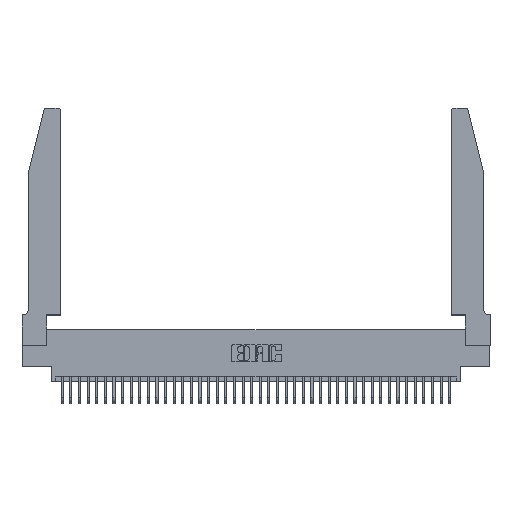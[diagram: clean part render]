
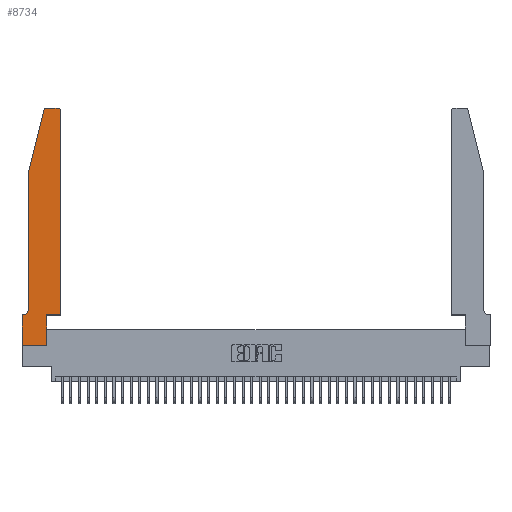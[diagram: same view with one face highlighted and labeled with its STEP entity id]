
A CAD part, top view. The second image highlights one B-rep face of the part: STEP entity #8734.
In plain terms, the highlighted planar face has unit normal (0, 0, 1).
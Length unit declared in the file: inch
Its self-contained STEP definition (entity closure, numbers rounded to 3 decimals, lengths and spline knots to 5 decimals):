
#609 = EDGE_CURVE ( 'NONE', #27823, #3113, #29730, .T. ) ;
#699 = CARTESIAN_POINT ( 'NONE',  ( 0.0055, 0.35, 0.37 ) ) ;
#1098 = DIRECTION ( 'NONE',  ( -1., 0., 0. ) ) ;
#1533 = CARTESIAN_POINT ( 'NONE',  ( 0.0755, 2., 0.37 ) ) ;
#1537 = VECTOR ( 'NONE', #41437, 39.37008 ) ;
#2118 = ORIENTED_EDGE ( 'NONE', *, *, #10758, .T. ) ;
#2122 = EDGE_CURVE ( 'NONE', #7781, #35161, #39446, .T. ) ;
#2533 = CARTESIAN_POINT ( 'NONE',  ( 0.2605, 2.75, 0.37 ) ) ;
#3113 = VERTEX_POINT ( 'NONE', #12753 ) ;
#3224 = CARTESIAN_POINT ( 'NONE',  ( 0.4505, 0.35, 0.37 ) ) ;
#3406 = AXIS2_PLACEMENT_3D ( 'NONE', #4545, #27411, #7865 ) ;
#3626 = EDGE_CURVE ( 'NONE', #7282, #7781, #19181, .T. ) ;
#4263 = ORIENTED_EDGE ( 'NONE', *, *, #15401, .T. ) ;
#4545 = CARTESIAN_POINT ( 'NONE',  ( 0.284, 2.72, 0.37 ) ) ;
#4593 = VERTEX_POINT ( 'NONE', #16736 ) ;
#4860 = EDGE_CURVE ( 'NONE', #18671, #27823, #8823, .T. ) ;
#5033 = EDGE_CURVE ( 'NONE', #14397, #7282, #27702, .T. ) ;
#5740 = AXIS2_PLACEMENT_3D ( 'NONE', #15810, #38343, #19061 ) ;
#5990 = LINE ( 'NONE', #33693, #39462 ) ;
#6028 = VERTEX_POINT ( 'NONE', #11312 ) ;
#6062 = LINE ( 'NONE', #2533, #21433 ) ;
#7217 = CARTESIAN_POINT ( 'NONE',  ( 0., 0., 0.37 ) ) ;
#7282 = VERTEX_POINT ( 'NONE', #34944 ) ;
#7315 = FACE_OUTER_BOUND ( 'NONE', #29174, .T. ) ;
#7396 = ORIENTED_EDGE ( 'NONE', *, *, #13555, .T. ) ;
#7781 = VERTEX_POINT ( 'NONE', #14451 ) ;
#7803 = VECTOR ( 'NONE', #40629, 39.37008 ) ;
#7865 = DIRECTION ( 'NONE',  ( 1., 0., 0. ) ) ;
#8544 = DIRECTION ( 'NONE',  ( 0., -1., 0. ) ) ;
#8734 = ADVANCED_FACE ( 'NONE', ( #7315 ), #35402, .T. ) ;
#8823 = LINE ( 'NONE', #1533, #7803 ) ;
#9170 = DIRECTION ( 'NONE',  ( 0., 1., 0. ) ) ;
#10758 = EDGE_CURVE ( 'NONE', #3113, #14397, #25016, .T. ) ;
#11088 = EDGE_CURVE ( 'NONE', #16154, #6028, #6062, .T. ) ;
#11312 = CARTESIAN_POINT ( 'NONE',  ( 0.284, 2.75, 0.37 ) ) ;
#11986 = EDGE_CURVE ( 'NONE', #35161, #25488, #5990, .T. ) ;
#12753 = CARTESIAN_POINT ( 'NONE',  ( 0.0755, 0.42, 0.37 ) ) ;
#13549 = ORIENTED_EDGE ( 'NONE', *, *, #2122, .T. ) ;
#13555 = EDGE_CURVE ( 'NONE', #4593, #16154, #34901, .T. ) ;
#14035 = AXIS2_PLACEMENT_3D ( 'NONE', #40077, #20820, #1098 ) ;
#14397 = VERTEX_POINT ( 'NONE', #699 ) ;
#14451 = CARTESIAN_POINT ( 'NONE',  ( 0., 0., 0.37 ) ) ;
#15401 = EDGE_CURVE ( 'NONE', #38449, #4593, #38650, .T. ) ;
#15714 = CARTESIAN_POINT ( 'NONE',  ( 0.0755, 0.35, 0.37 ) ) ;
#15810 = CARTESIAN_POINT ( 'NONE',  ( 0.4205, 2.72, 0.37 ) ) ;
#16079 = CARTESIAN_POINT ( 'NONE',  ( 0., 0.35, 0.37 ) ) ;
#16094 = CARTESIAN_POINT ( 'NONE',  ( 0.0755, 2., 0.37 ) ) ;
#16154 = VERTEX_POINT ( 'NONE', #23456 ) ;
#16559 = ORIENTED_EDGE ( 'NONE', *, *, #11088, .T. ) ;
#16736 = CARTESIAN_POINT ( 'NONE',  ( 0.4505, 2.72, 0.37 ) ) ;
#18094 = AXIS2_PLACEMENT_3D ( 'NONE', #16079, #41818, #22617 ) ;
#18112 = ORIENTED_EDGE ( 'NONE', *, *, #4860, .T. ) ;
#18192 = VECTOR ( 'NONE', #8544, 39.37008 ) ;
#18306 = CARTESIAN_POINT ( 'NONE',  ( 0., 0., 0.37 ) ) ;
#18671 = VERTEX_POINT ( 'NONE', #27500 ) ;
#19061 = DIRECTION ( 'NONE',  ( 1., 0., 0. ) ) ;
#19181 = LINE ( 'NONE', #18306, #18192 ) ;
#19639 = ORIENTED_EDGE ( 'NONE', *, *, #5033, .T. ) ;
#20488 = LINE ( 'NONE', #28219, #28115 ) ;
#20820 = DIRECTION ( 'NONE',  ( 0., 0., -1. ) ) ;
#20877 = DIRECTION ( 'NONE',  ( 0., 1., 0. ) ) ;
#21126 = VECTOR ( 'NONE', #35223, 39.37008 ) ;
#21341 = VECTOR ( 'NONE', #33766, 39.37008 ) ;
#21433 = VECTOR ( 'NONE', #38372, 39.37008 ) ;
#22617 = DIRECTION ( 'NONE',  ( 1., 0., 0. ) ) ;
#22714 = ORIENTED_EDGE ( 'NONE', *, *, #3626, .T. ) ;
#23456 = CARTESIAN_POINT ( 'NONE',  ( 0.4205, 2.75, 0.37 ) ) ;
#24703 = EDGE_CURVE ( 'NONE', #25488, #38449, #20488, .T. ) ;
#25016 = CIRCLE ( 'NONE', #14035, 0.07 ) ;
#25262 = ORIENTED_EDGE ( 'NONE', *, *, #24703, .T. ) ;
#25488 = VERTEX_POINT ( 'NONE', #35186 ) ;
#26239 = CARTESIAN_POINT ( 'NONE',  ( 0.2865, 0., 0.37 ) ) ;
#27411 = DIRECTION ( 'NONE',  ( 0., 0., 1. ) ) ;
#27500 = CARTESIAN_POINT ( 'NONE',  ( 0.25487, 2.72718, 0.37 ) ) ;
#27702 = LINE ( 'NONE', #15714, #1537 ) ;
#27823 = VERTEX_POINT ( 'NONE', #32200 ) ;
#28115 = VECTOR ( 'NONE', #31413, 39.37008 ) ;
#28219 = CARTESIAN_POINT ( 'NONE',  ( 0.4505, 0.35, 0.37 ) ) ;
#28720 = CARTESIAN_POINT ( 'NONE',  ( 0.4505, 0.35, 0.37 ) ) ;
#29174 = EDGE_LOOP ( 'NONE', ( #16559, #29219, #18112, #32746, #2118, #19639, #22714, #13549, #30795, #25262, #4263, #7396 ) ) ;
#29219 = ORIENTED_EDGE ( 'NONE', *, *, #38723, .T. ) ;
#29730 = LINE ( 'NONE', #16094, #21126 ) ;
#30795 = ORIENTED_EDGE ( 'NONE', *, *, #11986, .T. ) ;
#31413 = DIRECTION ( 'NONE',  ( 1., 0., 0. ) ) ;
#32200 = CARTESIAN_POINT ( 'NONE',  ( 0.0755, 2., 0.37 ) ) ;
#32746 = ORIENTED_EDGE ( 'NONE', *, *, #609, .T. ) ;
#33693 = CARTESIAN_POINT ( 'NONE',  ( 0.2865, 0.35, 0.37 ) ) ;
#33766 = DIRECTION ( 'NONE',  ( 1., 0., 0. ) ) ;
#34901 = CIRCLE ( 'NONE', #5740, 0.03 ) ;
#34944 = CARTESIAN_POINT ( 'NONE',  ( 0., 0.35, 0.37 ) ) ;
#35161 = VERTEX_POINT ( 'NONE', #26239 ) ;
#35186 = CARTESIAN_POINT ( 'NONE',  ( 0.2865, 0.35, 0.37 ) ) ;
#35223 = DIRECTION ( 'NONE',  ( 0., -1., 0. ) ) ;
#35305 = CIRCLE ( 'NONE', #3406, 0.03 ) ;
#35402 = PLANE ( 'NONE',  #18094 ) ;
#38343 = DIRECTION ( 'NONE',  ( 0., 0., 1. ) ) ;
#38372 = DIRECTION ( 'NONE',  ( -1., 0., 0. ) ) ;
#38449 = VERTEX_POINT ( 'NONE', #3224 ) ;
#38650 = LINE ( 'NONE', #28720, #41653 ) ;
#38723 = EDGE_CURVE ( 'NONE', #6028, #18671, #35305, .T. ) ;
#39446 = LINE ( 'NONE', #7217, #21341 ) ;
#39462 = VECTOR ( 'NONE', #20877, 39.37008 ) ;
#40077 = CARTESIAN_POINT ( 'NONE',  ( 0.0055, 0.42, 0.37 ) ) ;
#40629 = DIRECTION ( 'NONE',  ( -0.239, -0.971, 0. ) ) ;
#41437 = DIRECTION ( 'NONE',  ( -1., 0., 0. ) ) ;
#41653 = VECTOR ( 'NONE', #9170, 39.37008 ) ;
#41818 = DIRECTION ( 'NONE',  ( 0., 0., 1. ) ) ;
